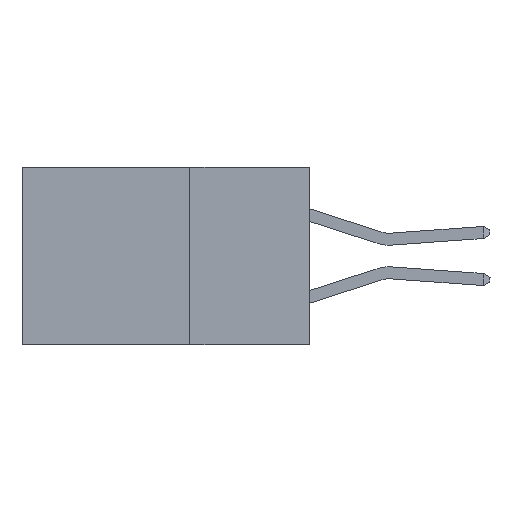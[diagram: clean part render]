
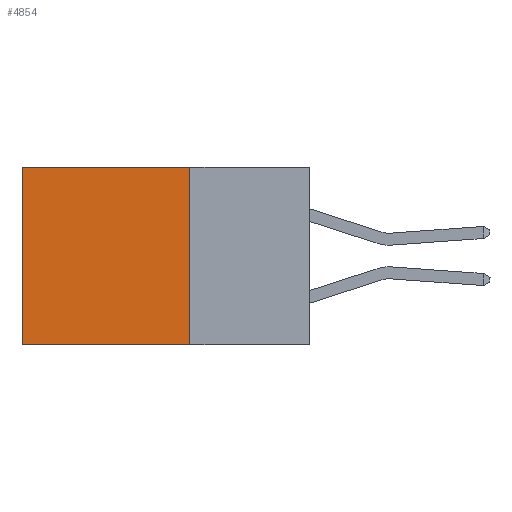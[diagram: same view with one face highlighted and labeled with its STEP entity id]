
A CAD part, left-side view. The second image highlights one B-rep face of the part: STEP entity #4854.
In plain terms, the highlighted planar face has unit normal (-1, 0, 0).
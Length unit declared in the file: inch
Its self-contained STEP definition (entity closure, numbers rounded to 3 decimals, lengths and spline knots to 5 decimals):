
#92 = ORIENTED_EDGE ( 'NONE', *, *, #800, .T. ) ;
#404 = CARTESIAN_POINT ( 'NONE',  ( 0.298, 0.25, 0. ) ) ;
#800 = EDGE_CURVE ( 'NONE', #2399, #10284, #2371, .T. ) ;
#850 = CARTESIAN_POINT ( 'NONE',  ( 0.298, 0.25, 0. ) ) ;
#899 = VECTOR ( 'NONE', #1864, 39.37008 ) ;
#1127 = DIRECTION ( 'NONE',  ( 0., 1., 0. ) ) ;
#1159 = PLANE ( 'NONE',  #9291 ) ;
#1425 = DIRECTION ( 'NONE',  ( 0., 1., 0. ) ) ;
#1452 = DIRECTION ( 'NONE',  ( 0., 0., -1. ) ) ;
#1864 = DIRECTION ( 'NONE',  ( 0., 0., -1. ) ) ;
#1904 = VECTOR ( 'NONE', #1127, 39.37008 ) ;
#2371 = LINE ( 'NONE', #10566, #4301 ) ;
#2399 = VERTEX_POINT ( 'NONE', #4910 ) ;
#2821 = VERTEX_POINT ( 'NONE', #7988 ) ;
#3071 = CARTESIAN_POINT ( 'NONE',  ( 0.298, 0.25, 0. ) ) ;
#3171 = EDGE_LOOP ( 'NONE', ( #92, #9251, #7153, #5184 ) ) ;
#3242 = EDGE_CURVE ( 'NONE', #4424, #2821, #6869, .T. ) ;
#4100 = EDGE_CURVE ( 'NONE', #4424, #2399, #9433, .T. ) ;
#4293 = CARTESIAN_POINT ( 'NONE',  ( 0.298, 0.25, 0. ) ) ;
#4301 = VECTOR ( 'NONE', #1452, 39.37008 ) ;
#4417 = CARTESIAN_POINT ( 'NONE',  ( 0.298, 0.25, -0.37 ) ) ;
#4424 = VERTEX_POINT ( 'NONE', #850 ) ;
#4808 = EDGE_CURVE ( 'NONE', #2821, #10284, #9170, .T. ) ;
#4854 = ADVANCED_FACE ( 'NONE', ( #7108 ), #1159, .F. ) ;
#4910 = CARTESIAN_POINT ( 'NONE',  ( 0.298, 0.6, 0. ) ) ;
#5184 = ORIENTED_EDGE ( 'NONE', *, *, #4100, .T. ) ;
#6186 = DIRECTION ( 'NONE',  ( 1., 0., 0. ) ) ;
#6869 = LINE ( 'NONE', #4293, #899 ) ;
#7108 = FACE_OUTER_BOUND ( 'NONE', #3171, .T. ) ;
#7153 = ORIENTED_EDGE ( 'NONE', *, *, #3242, .F. ) ;
#7766 = VECTOR ( 'NONE', #1425, 39.37008 ) ;
#7988 = CARTESIAN_POINT ( 'NONE',  ( 0.298, 0.25, -0.37 ) ) ;
#8698 = DIRECTION ( 'NONE',  ( 0., 0., -1. ) ) ;
#9170 = LINE ( 'NONE', #4417, #1904 ) ;
#9251 = ORIENTED_EDGE ( 'NONE', *, *, #4808, .F. ) ;
#9291 = AXIS2_PLACEMENT_3D ( 'NONE', #404, #6186, #8698 ) ;
#9433 = LINE ( 'NONE', #3071, #7766 ) ;
#9654 = CARTESIAN_POINT ( 'NONE',  ( 0.298, 0.6, -0.37 ) ) ;
#10284 = VERTEX_POINT ( 'NONE', #9654 ) ;
#10566 = CARTESIAN_POINT ( 'NONE',  ( 0.298, 0.6, 0. ) ) ;
